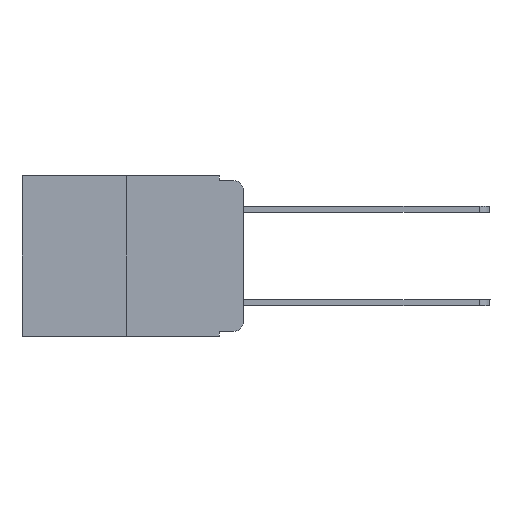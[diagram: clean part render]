
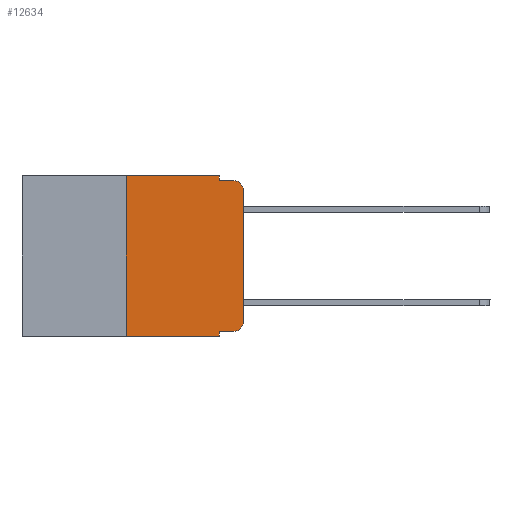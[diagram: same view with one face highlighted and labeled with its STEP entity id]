
A CAD part, left-side view. The second image highlights one B-rep face of the part: STEP entity #12634.
In plain terms, the highlighted planar face has unit normal (-1, 0, 0).
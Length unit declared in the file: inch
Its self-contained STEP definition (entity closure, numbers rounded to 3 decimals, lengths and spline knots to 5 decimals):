
#117 = DIRECTION ( 'NONE',  ( 0., -1., 0. ) ) ;
#143 = CARTESIAN_POINT ( 'NONE',  ( 0., 0.02, -0.313 ) ) ;
#476 = EDGE_CURVE ( 'NONE', #14060, #8134, #8036, .T. ) ;
#619 = EDGE_CURVE ( 'NONE', #3406, #14060, #10566, .T. ) ;
#707 = CARTESIAN_POINT ( 'NONE',  ( 0., 0.02, -0.01 ) ) ;
#738 = VERTEX_POINT ( 'NONE', #7154 ) ;
#797 = CARTESIAN_POINT ( 'NONE',  ( 0., 0.473, 0. ) ) ;
#1082 = CARTESIAN_POINT ( 'NONE',  ( 0., 0.051, -0.333 ) ) ;
#1100 = CARTESIAN_POINT ( 'NONE',  ( 0., 0.051, -0.333 ) ) ;
#1105 = VECTOR ( 'NONE', #117, 39.37008 ) ;
#1172 = DIRECTION ( 'NONE',  ( 0., -1., 0. ) ) ;
#1347 = CIRCLE ( 'NONE', #10601, 0.02 ) ;
#1451 = DIRECTION ( 'NONE',  ( 0., 0., -1. ) ) ;
#1531 = CARTESIAN_POINT ( 'NONE',  ( 0., 0.25, -0.343 ) ) ;
#1605 = PLANE ( 'NONE',  #6772 ) ;
#1856 = VERTEX_POINT ( 'NONE', #8368 ) ;
#2062 = VECTOR ( 'NONE', #7828, 39.37008 ) ;
#2131 = DIRECTION ( 'NONE',  ( -1., 0., 0. ) ) ;
#2292 = ORIENTED_EDGE ( 'NONE', *, *, #14496, .F. ) ;
#2312 = ORIENTED_EDGE ( 'NONE', *, *, #619, .T. ) ;
#2411 = LINE ( 'NONE', #7442, #8997 ) ;
#2469 = DIRECTION ( 'NONE',  ( -1., 0., 0. ) ) ;
#2471 = VERTEX_POINT ( 'NONE', #6736 ) ;
#2641 = DIRECTION ( 'NONE',  ( 0., -1., 0. ) ) ;
#3406 = VERTEX_POINT ( 'NONE', #15065 ) ;
#3576 = DIRECTION ( 'NONE',  ( 0., 0., 1. ) ) ;
#3659 = AXIS2_PLACEMENT_3D ( 'NONE', #5839, #2131, #12951 ) ;
#3867 = EDGE_CURVE ( 'NONE', #11245, #15286, #2411, .T. ) ;
#4380 = VERTEX_POINT ( 'NONE', #12920 ) ;
#4416 = ORIENTED_EDGE ( 'NONE', *, *, #11725, .T. ) ;
#4507 = FACE_OUTER_BOUND ( 'NONE', #12484, .T. ) ;
#4520 = VECTOR ( 'NONE', #1172, 39.37008 ) ;
#4776 = CARTESIAN_POINT ( 'NONE',  ( 0., 0., 0. ) ) ;
#5133 = ORIENTED_EDGE ( 'NONE', *, *, #3867, .T. ) ;
#5208 = VECTOR ( 'NONE', #1451, 39.37008 ) ;
#5645 = VERTEX_POINT ( 'NONE', #1082 ) ;
#5839 = CARTESIAN_POINT ( 'NONE',  ( 0., 0.02, -0.03 ) ) ;
#6031 = VECTOR ( 'NONE', #11656, 39.37008 ) ;
#6245 = LINE ( 'NONE', #6510, #8302 ) ;
#6510 = CARTESIAN_POINT ( 'NONE',  ( 0., 0.051, 0. ) ) ;
#6736 = CARTESIAN_POINT ( 'NONE',  ( 0., 0.25, 0. ) ) ;
#6772 = AXIS2_PLACEMENT_3D ( 'NONE', #12397, #9175, #10014 ) ;
#6851 = ORIENTED_EDGE ( 'NONE', *, *, #12306, .F. ) ;
#7154 = CARTESIAN_POINT ( 'NONE',  ( 0., 0.051, -0.01 ) ) ;
#7350 = ORIENTED_EDGE ( 'NONE', *, *, #10103, .F. ) ;
#7442 = CARTESIAN_POINT ( 'NONE',  ( 0., 0.473, -0.343 ) ) ;
#7637 = ORIENTED_EDGE ( 'NONE', *, *, #11949, .F. ) ;
#7828 = DIRECTION ( 'NONE',  ( 0., 0., 1. ) ) ;
#7918 = CARTESIAN_POINT ( 'NONE',  ( 0., 0.25, 0. ) ) ;
#8036 = CIRCLE ( 'NONE', #3659, 0.02 ) ;
#8134 = VERTEX_POINT ( 'NONE', #707 ) ;
#8302 = VECTOR ( 'NONE', #11126, 39.37008 ) ;
#8368 = CARTESIAN_POINT ( 'NONE',  ( 0., 0.051, 0. ) ) ;
#8766 = CARTESIAN_POINT ( 'NONE',  ( 0., 0.051, 0. ) ) ;
#8997 = VECTOR ( 'NONE', #2641, 39.37008 ) ;
#9035 = LINE ( 'NONE', #797, #6031 ) ;
#9170 = LINE ( 'NONE', #8766, #5208 ) ;
#9175 = DIRECTION ( 'NONE',  ( 1., 0., 0. ) ) ;
#9452 = ORIENTED_EDGE ( 'NONE', *, *, #12913, .T. ) ;
#9856 = ORIENTED_EDGE ( 'NONE', *, *, #476, .T. ) ;
#10001 = ORIENTED_EDGE ( 'NONE', *, *, #12676, .F. ) ;
#10014 = DIRECTION ( 'NONE',  ( 0., 0., -1. ) ) ;
#10103 = EDGE_CURVE ( 'NONE', #11245, #2471, #14424, .T. ) ;
#10195 = VECTOR ( 'NONE', #3576, 39.37008 ) ;
#10566 = LINE ( 'NONE', #4776, #10195 ) ;
#10601 = AXIS2_PLACEMENT_3D ( 'NONE', #143, #2469, #14411 ) ;
#11126 = DIRECTION ( 'NONE',  ( 0., 0., -1. ) ) ;
#11245 = VERTEX_POINT ( 'NONE', #1531 ) ;
#11618 = LINE ( 'NONE', #1100, #1105 ) ;
#11656 = DIRECTION ( 'NONE',  ( 0., -1., 0. ) ) ;
#11725 = EDGE_CURVE ( 'NONE', #4380, #3406, #1347, .T. ) ;
#11949 = EDGE_CURVE ( 'NONE', #5645, #15286, #6245, .T. ) ;
#12306 = EDGE_CURVE ( 'NONE', #738, #8134, #13130, .T. ) ;
#12397 = CARTESIAN_POINT ( 'NONE',  ( 0., 0.473, 0. ) ) ;
#12484 = EDGE_LOOP ( 'NONE', ( #2312, #9856, #6851, #2292, #10001, #7350, #5133, #7637, #9452, #4416 ) ) ;
#12634 = ADVANCED_FACE ( 'NONE', ( #4507 ), #1605, .F. ) ;
#12676 = EDGE_CURVE ( 'NONE', #2471, #1856, #9035, .T. ) ;
#12913 = EDGE_CURVE ( 'NONE', #5645, #4380, #11618, .T. ) ;
#12920 = CARTESIAN_POINT ( 'NONE',  ( 0., 0.02, -0.333 ) ) ;
#12951 = DIRECTION ( 'NONE',  ( 0., 0., -1. ) ) ;
#13082 = CARTESIAN_POINT ( 'NONE',  ( 0., 0.051, -0.01 ) ) ;
#13130 = LINE ( 'NONE', #13082, #4520 ) ;
#13807 = CARTESIAN_POINT ( 'NONE',  ( 0., 0.051, -0.343 ) ) ;
#13942 = CARTESIAN_POINT ( 'NONE',  ( 0., 0., -0.03 ) ) ;
#14060 = VERTEX_POINT ( 'NONE', #13942 ) ;
#14411 = DIRECTION ( 'NONE',  ( 0., 0., -1. ) ) ;
#14424 = LINE ( 'NONE', #7918, #2062 ) ;
#14496 = EDGE_CURVE ( 'NONE', #1856, #738, #9170, .T. ) ;
#15065 = CARTESIAN_POINT ( 'NONE',  ( 0., 0., -0.313 ) ) ;
#15286 = VERTEX_POINT ( 'NONE', #13807 ) ;
